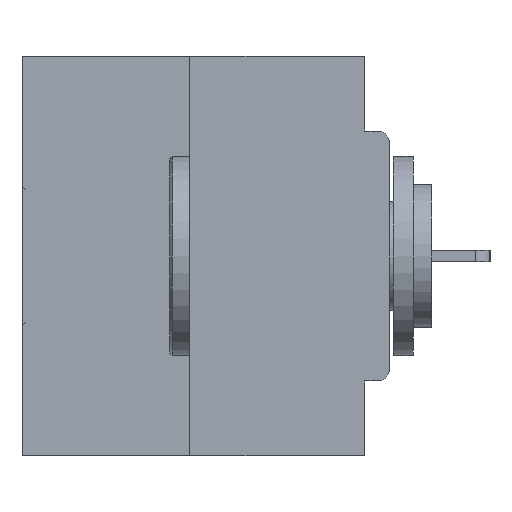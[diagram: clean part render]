
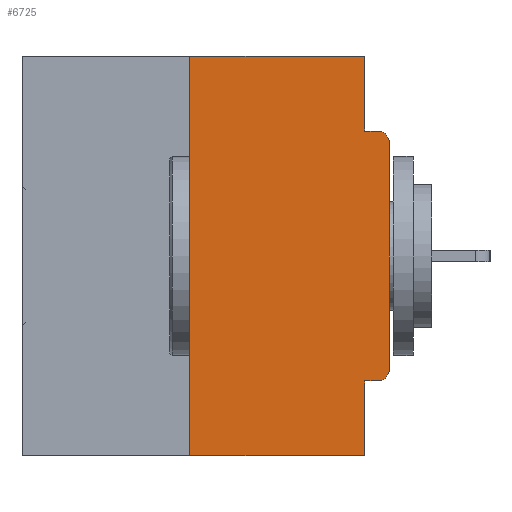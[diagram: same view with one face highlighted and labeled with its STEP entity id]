
A CAD part, left-side view. The second image highlights one B-rep face of the part: STEP entity #6725.
In plain terms, the highlighted planar face has unit normal (-1, 0, 0).
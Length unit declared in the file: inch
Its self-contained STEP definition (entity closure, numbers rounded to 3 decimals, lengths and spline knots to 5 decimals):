
#800 = CARTESIAN_POINT ( 'NONE',  ( 0., 0.031, -0.4065 ) ) ;
#916 = EDGE_LOOP ( 'NONE', ( #14543, #1005, #30476, #31436, #19242, #20596, #3208, #1183, #14608, #3947 ) ) ;
#1005 = ORIENTED_EDGE ( 'NONE', *, *, #18990, .F. ) ;
#1044 = CARTESIAN_POINT ( 'NONE',  ( 0., 0.031, 0. ) ) ;
#1049 = LINE ( 'NONE', #28614, #6937 ) ;
#1183 = ORIENTED_EDGE ( 'NONE', *, *, #15549, .T. ) ;
#1237 = DIRECTION ( 'NONE',  ( 0., 0., -1. ) ) ;
#1346 = EDGE_CURVE ( 'NONE', #3376, #12305, #36892, .T. ) ;
#2409 = DIRECTION ( 'NONE',  ( 0., 0., 1. ) ) ;
#2916 = VERTEX_POINT ( 'NONE', #30483 ) ;
#3208 = ORIENTED_EDGE ( 'NONE', *, *, #19724, .T. ) ;
#3376 = VERTEX_POINT ( 'NONE', #13484 ) ;
#3864 = CARTESIAN_POINT ( 'NONE',  ( 0., 0.031, -0.5 ) ) ;
#3947 = ORIENTED_EDGE ( 'NONE', *, *, #36764, .F. ) ;
#4465 = DIRECTION ( 'NONE',  ( 0., 1., 0. ) ) ;
#4831 = CARTESIAN_POINT ( 'NONE',  ( 0., 0., -0.4065 ) ) ;
#5187 = CARTESIAN_POINT ( 'NONE',  ( 0., 0., 0. ) ) ;
#5969 = AXIS2_PLACEMENT_3D ( 'NONE', #33560, #16465, #36359 ) ;
#6449 = VECTOR ( 'NONE', #2409, 39.37008 ) ;
#6523 = VERTEX_POINT ( 'NONE', #19545 ) ;
#6722 = DIRECTION ( 'NONE',  ( 0., 0., -1. ) ) ;
#6725 = ADVANCED_FACE ( 'NONE', ( #30099 ), #8982, .F. ) ;
#6937 = VECTOR ( 'NONE', #25934, 39.37008 ) ;
#7315 = VECTOR ( 'NONE', #6722, 39.37008 ) ;
#7353 = LINE ( 'NONE', #5187, #6449 ) ;
#8234 = LINE ( 'NONE', #3864, #7315 ) ;
#8982 = PLANE ( 'NONE',  #25548 ) ;
#9027 = LINE ( 'NONE', #33453, #30837 ) ;
#10221 = VECTOR ( 'NONE', #20240, 39.37008 ) ;
#10880 = CARTESIAN_POINT ( 'NONE',  ( 0., 0.25, -0.5 ) ) ;
#11905 = VERTEX_POINT ( 'NONE', #18702 ) ;
#11972 = LINE ( 'NONE', #20165, #33753 ) ;
#12305 = VERTEX_POINT ( 'NONE', #800 ) ;
#12358 = VERTEX_POINT ( 'NONE', #1044 ) ;
#13185 = VERTEX_POINT ( 'NONE', #19140 ) ;
#13484 = CARTESIAN_POINT ( 'NONE',  ( 0., 0.015, -0.4065 ) ) ;
#13548 = DIRECTION ( 'NONE',  ( 0., -1., 0. ) ) ;
#13850 = CARTESIAN_POINT ( 'NONE',  ( 0., 0.031, 0. ) ) ;
#14543 = ORIENTED_EDGE ( 'NONE', *, *, #30895, .F. ) ;
#14608 = ORIENTED_EDGE ( 'NONE', *, *, #21446, .F. ) ;
#14624 = CARTESIAN_POINT ( 'NONE',  ( 0., 0.015, -0.0935 ) ) ;
#14640 = DIRECTION ( 'NONE',  ( 1., 0., 0. ) ) ;
#15549 = EDGE_CURVE ( 'NONE', #13185, #21701, #36277, .T. ) ;
#16465 = DIRECTION ( 'NONE',  ( -1., 0., 0. ) ) ;
#17269 = EDGE_CURVE ( 'NONE', #12305, #11905, #8234, .T. ) ;
#17435 = VECTOR ( 'NONE', #36554, 39.37008 ) ;
#17690 = LINE ( 'NONE', #28944, #10221 ) ;
#17754 = EDGE_CURVE ( 'NONE', #36748, #11905, #11972, .T. ) ;
#18356 = DIRECTION ( 'NONE',  ( -1., 0., 0. ) ) ;
#18702 = CARTESIAN_POINT ( 'NONE',  ( 0., 0.031, -0.5 ) ) ;
#18990 = EDGE_CURVE ( 'NONE', #36748, #24718, #1049, .T. ) ;
#19140 = CARTESIAN_POINT ( 'NONE',  ( 0., 0., -0.1085 ) ) ;
#19242 = ORIENTED_EDGE ( 'NONE', *, *, #1346, .F. ) ;
#19254 = LINE ( 'NONE', #13850, #17435 ) ;
#19545 = CARTESIAN_POINT ( 'NONE',  ( 0., 0.031, -0.0935 ) ) ;
#19724 = EDGE_CURVE ( 'NONE', #2916, #13185, #7353, .T. ) ;
#20165 = CARTESIAN_POINT ( 'NONE',  ( 0., 0.46, -0.5 ) ) ;
#20240 = DIRECTION ( 'NONE',  ( 0., -1., 0. ) ) ;
#20596 = ORIENTED_EDGE ( 'NONE', *, *, #35821, .T. ) ;
#20970 = VECTOR ( 'NONE', #4465, 39.37008 ) ;
#21446 = EDGE_CURVE ( 'NONE', #6523, #21701, #9027, .T. ) ;
#21701 = VERTEX_POINT ( 'NONE', #14624 ) ;
#23090 = DIRECTION ( 'NONE',  ( 0., -1., 0. ) ) ;
#24718 = VERTEX_POINT ( 'NONE', #26065 ) ;
#25548 = AXIS2_PLACEMENT_3D ( 'NONE', #28932, #14640, #34545 ) ;
#25934 = DIRECTION ( 'NONE',  ( 0., 0., 1. ) ) ;
#26065 = CARTESIAN_POINT ( 'NONE',  ( 0., 0.25, 0. ) ) ;
#28614 = CARTESIAN_POINT ( 'NONE',  ( 0., 0.25, 0. ) ) ;
#28932 = CARTESIAN_POINT ( 'NONE',  ( 0., 0.46, 0. ) ) ;
#28944 = CARTESIAN_POINT ( 'NONE',  ( 0., 0.46, 0. ) ) ;
#30083 = AXIS2_PLACEMENT_3D ( 'NONE', #35385, #18356, #1237 ) ;
#30099 = FACE_OUTER_BOUND ( 'NONE', #916, .T. ) ;
#30476 = ORIENTED_EDGE ( 'NONE', *, *, #17754, .T. ) ;
#30483 = CARTESIAN_POINT ( 'NONE',  ( 0., 0., -0.3915 ) ) ;
#30837 = VECTOR ( 'NONE', #13548, 39.37008 ) ;
#30895 = EDGE_CURVE ( 'NONE', #24718, #12358, #17690, .T. ) ;
#31436 = ORIENTED_EDGE ( 'NONE', *, *, #17269, .F. ) ;
#33453 = CARTESIAN_POINT ( 'NONE',  ( 0., 0., -0.0935 ) ) ;
#33560 = CARTESIAN_POINT ( 'NONE',  ( 0., 0.015, -0.3915 ) ) ;
#33753 = VECTOR ( 'NONE', #23090, 39.37008 ) ;
#34545 = DIRECTION ( 'NONE',  ( 0., 0., -1. ) ) ;
#35171 = CIRCLE ( 'NONE', #5969, 0.015 ) ;
#35385 = CARTESIAN_POINT ( 'NONE',  ( 0., 0.015, -0.1085 ) ) ;
#35821 = EDGE_CURVE ( 'NONE', #3376, #2916, #35171, .T. ) ;
#36277 = CIRCLE ( 'NONE', #30083, 0.015 ) ;
#36359 = DIRECTION ( 'NONE',  ( 0., 0., -1. ) ) ;
#36554 = DIRECTION ( 'NONE',  ( 0., 0., -1. ) ) ;
#36748 = VERTEX_POINT ( 'NONE', #10880 ) ;
#36764 = EDGE_CURVE ( 'NONE', #12358, #6523, #19254, .T. ) ;
#36892 = LINE ( 'NONE', #4831, #20970 ) ;
